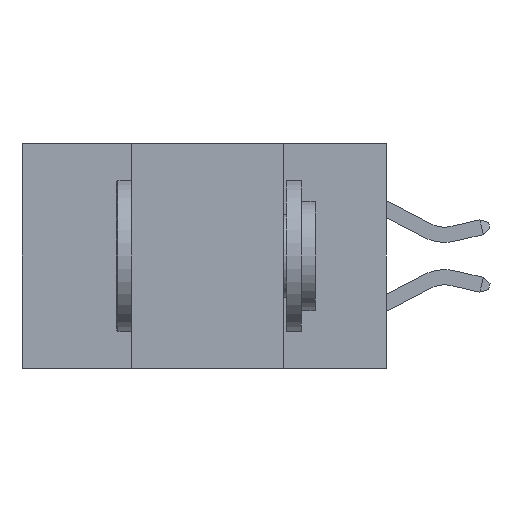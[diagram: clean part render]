
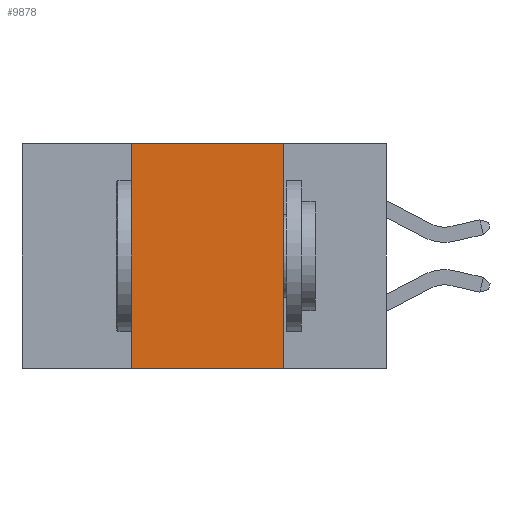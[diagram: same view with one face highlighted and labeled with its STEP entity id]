
A CAD part, left-side view. The second image highlights one B-rep face of the part: STEP entity #9878.
In plain terms, the highlighted planar face has unit normal (-1, 0, 0).
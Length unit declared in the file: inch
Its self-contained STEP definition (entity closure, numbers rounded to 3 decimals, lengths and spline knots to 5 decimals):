
#203 = CARTESIAN_POINT ( 'NONE',  ( 0., 0.42, 0. ) ) ;
#231 = EDGE_CURVE ( 'NONE', #12192, #12407, #2912, .T. ) ;
#253 = CARTESIAN_POINT ( 'NONE',  ( 0., 0.42, -0.37 ) ) ;
#341 = CARTESIAN_POINT ( 'NONE',  ( 0., 0.6, 0. ) ) ;
#655 = CARTESIAN_POINT ( 'NONE',  ( 0., 0.6, 0. ) ) ;
#709 = ORIENTED_EDGE ( 'NONE', *, *, #231, .F. ) ;
#1215 = EDGE_CURVE ( 'NONE', #12407, #4255, #3853, .T. ) ;
#1261 = CARTESIAN_POINT ( 'NONE',  ( 0., 0.42, -0.37 ) ) ;
#1445 = DIRECTION ( 'NONE',  ( 0., -1., 0. ) ) ;
#1520 = LINE ( 'NONE', #1261, #11329 ) ;
#2912 = LINE ( 'NONE', #655, #15199 ) ;
#3818 = ORIENTED_EDGE ( 'NONE', *, *, #1215, .F. ) ;
#3853 = LINE ( 'NONE', #7060, #9906 ) ;
#4200 = ORIENTED_EDGE ( 'NONE', *, *, #15217, .F. ) ;
#4255 = VERTEX_POINT ( 'NONE', #12652 ) ;
#5343 = VERTEX_POINT ( 'NONE', #253 ) ;
#6281 = DIRECTION ( 'NONE',  ( 0., 0., 1. ) ) ;
#6449 = CARTESIAN_POINT ( 'NONE',  ( 0., 0.6, -0.37 ) ) ;
#6757 = FACE_OUTER_BOUND ( 'NONE', #7487, .T. ) ;
#7060 = CARTESIAN_POINT ( 'NONE',  ( 0., 0.17, -0.37 ) ) ;
#7487 = EDGE_LOOP ( 'NONE', ( #3818, #709, #4200, #10633 ) ) ;
#7600 = DIRECTION ( 'NONE',  ( 0., 0., -1. ) ) ;
#9649 = VECTOR ( 'NONE', #1445, 39.37008 ) ;
#9878 = ADVANCED_FACE ( 'NONE', ( #6757 ), #13444, .F. ) ;
#9906 = VECTOR ( 'NONE', #7600, 39.37008 ) ;
#9967 = DIRECTION ( 'NONE',  ( 0., -1., 0. ) ) ;
#10633 = ORIENTED_EDGE ( 'NONE', *, *, #14518, .T. ) ;
#10796 = CARTESIAN_POINT ( 'NONE',  ( 0., 0.17, 0. ) ) ;
#11329 = VECTOR ( 'NONE', #6281, 39.37008 ) ;
#12192 = VERTEX_POINT ( 'NONE', #203 ) ;
#12407 = VERTEX_POINT ( 'NONE', #10796 ) ;
#12494 = LINE ( 'NONE', #6449, #9649 ) ;
#12652 = CARTESIAN_POINT ( 'NONE',  ( 0., 0.17, -0.37 ) ) ;
#13414 = DIRECTION ( 'NONE',  ( 0., 0., -1. ) ) ;
#13428 = DIRECTION ( 'NONE',  ( 1., 0., 0. ) ) ;
#13444 = PLANE ( 'NONE',  #14803 ) ;
#14518 = EDGE_CURVE ( 'NONE', #5343, #4255, #12494, .T. ) ;
#14803 = AXIS2_PLACEMENT_3D ( 'NONE', #341, #13428, #13414 ) ;
#15199 = VECTOR ( 'NONE', #9967, 39.37008 ) ;
#15217 = EDGE_CURVE ( 'NONE', #5343, #12192, #1520, .T. ) ;
